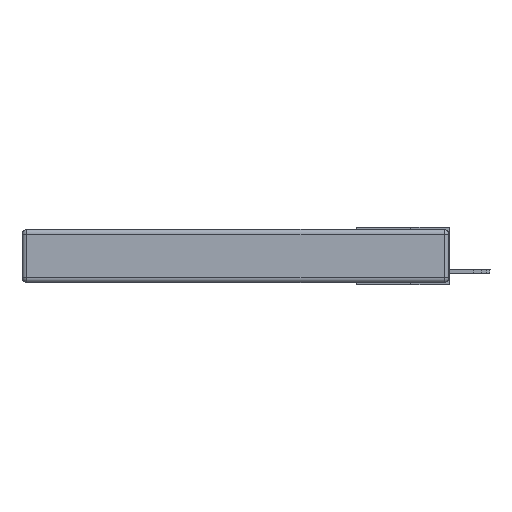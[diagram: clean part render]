
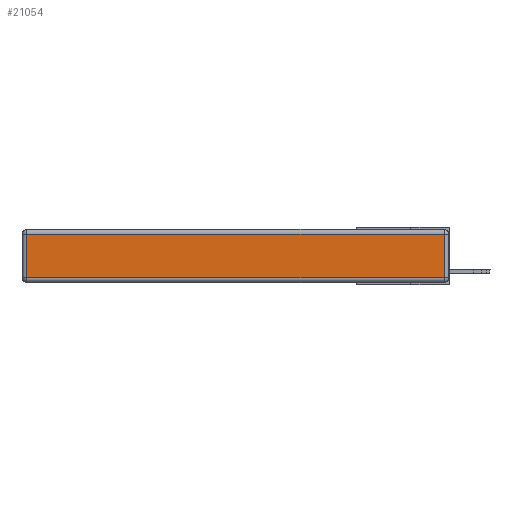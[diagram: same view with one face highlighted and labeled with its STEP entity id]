
A CAD part, left-side view. The second image highlights one B-rep face of the part: STEP entity #21054.
In plain terms, the highlighted planar face has unit normal (-1, 0, 0).
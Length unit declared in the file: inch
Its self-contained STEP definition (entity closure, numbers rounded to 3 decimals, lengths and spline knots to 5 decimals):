
#737 = ORIENTED_EDGE ( 'NONE', *, *, #20044, .T. ) ;
#951 = PLANE ( 'NONE',  #10669 ) ;
#1904 = VERTEX_POINT ( 'NONE', #11691 ) ;
#2972 = DIRECTION ( 'NONE',  ( 0., 0., 1. ) ) ;
#3651 = CARTESIAN_POINT ( 'NONE',  ( 0., 0., -0.313 ) ) ;
#4143 = EDGE_CURVE ( 'NONE', #8781, #16929, #13011, .T. ) ;
#4946 = DIRECTION ( 'NONE',  ( 0., 0., 1. ) ) ;
#5888 = CARTESIAN_POINT ( 'NONE',  ( 0., 2.72, -0.343 ) ) ;
#5936 = EDGE_CURVE ( 'NONE', #17684, #1904, #12943, .T. ) ;
#6545 = VECTOR ( 'NONE', #23721, 39.37008 ) ;
#7538 = DIRECTION ( 'NONE',  ( 0., -1., 0. ) ) ;
#7809 = CARTESIAN_POINT ( 'NONE',  ( 0., 0.03, -0.313 ) ) ;
#8781 = VERTEX_POINT ( 'NONE', #15335 ) ;
#8954 = LINE ( 'NONE', #22953, #18616 ) ;
#10669 = AXIS2_PLACEMENT_3D ( 'NONE', #10992, #12995, #2972 ) ;
#10948 = LINE ( 'NONE', #5888, #6545 ) ;
#10992 = CARTESIAN_POINT ( 'NONE',  ( 0., 0., -0.343 ) ) ;
#11691 = CARTESIAN_POINT ( 'NONE',  ( 0., 2.72, -0.03 ) ) ;
#12943 = LINE ( 'NONE', #22112, #16074 ) ;
#12995 = DIRECTION ( 'NONE',  ( -1., 0., 0. ) ) ;
#13011 = LINE ( 'NONE', #3651, #23613 ) ;
#15335 = CARTESIAN_POINT ( 'NONE',  ( 0., 2.72, -0.313 ) ) ;
#15611 = ORIENTED_EDGE ( 'NONE', *, *, #23784, .T. ) ;
#16074 = VECTOR ( 'NONE', #19770, 39.37008 ) ;
#16878 = CARTESIAN_POINT ( 'NONE',  ( 0., 0.03, -0.03 ) ) ;
#16929 = VERTEX_POINT ( 'NONE', #7809 ) ;
#17684 = VERTEX_POINT ( 'NONE', #16878 ) ;
#18616 = VECTOR ( 'NONE', #4946, 39.37008 ) ;
#19770 = DIRECTION ( 'NONE',  ( 0., 1., 0. ) ) ;
#20044 = EDGE_CURVE ( 'NONE', #16929, #17684, #8954, .T. ) ;
#21054 = ADVANCED_FACE ( 'NONE', ( #25412 ), #951, .T. ) ;
#21703 = ORIENTED_EDGE ( 'NONE', *, *, #4143, .T. ) ;
#22112 = CARTESIAN_POINT ( 'NONE',  ( 0., 2.75, -0.03 ) ) ;
#22953 = CARTESIAN_POINT ( 'NONE',  ( 0., 0.03, -0.343 ) ) ;
#23613 = VECTOR ( 'NONE', #7538, 39.37008 ) ;
#23721 = DIRECTION ( 'NONE',  ( 0., 0., -1. ) ) ;
#23784 = EDGE_CURVE ( 'NONE', #1904, #8781, #10948, .T. ) ;
#24102 = EDGE_LOOP ( 'NONE', ( #21703, #737, #25321, #15611 ) ) ;
#25321 = ORIENTED_EDGE ( 'NONE', *, *, #5936, .T. ) ;
#25412 = FACE_OUTER_BOUND ( 'NONE', #24102, .T. ) ;
